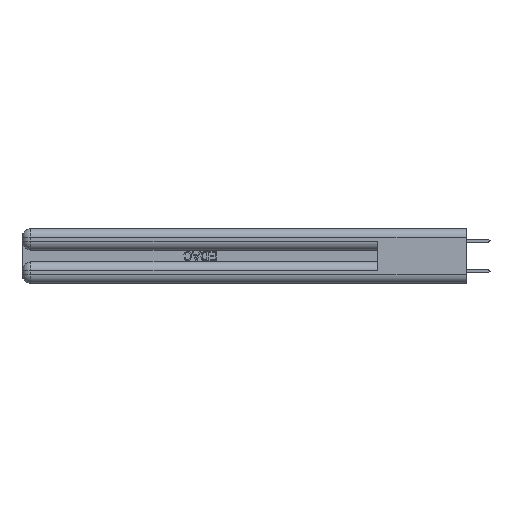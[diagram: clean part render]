
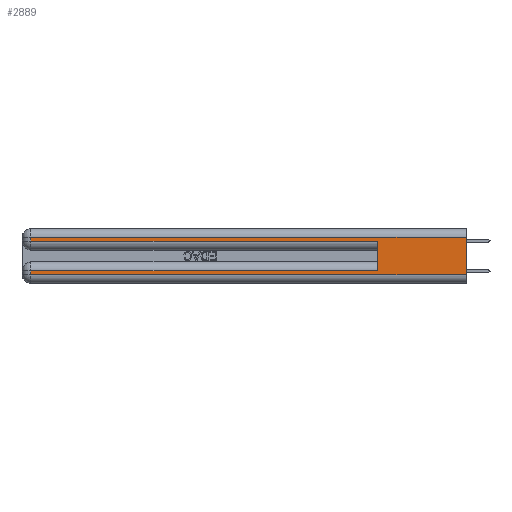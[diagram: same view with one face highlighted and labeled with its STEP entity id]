
A CAD part, left-side view. The second image highlights one B-rep face of the part: STEP entity #2889.
In plain terms, the highlighted planar face has unit normal (-1, 0, 0).
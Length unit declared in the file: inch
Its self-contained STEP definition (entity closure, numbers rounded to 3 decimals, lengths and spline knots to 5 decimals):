
#321 = CARTESIAN_POINT ( 'NONE',  ( 0., 0., 0.31 ) ) ;
#452 = VECTOR ( 'NONE', #42532, 39.37008 ) ;
#540 = DIRECTION ( 'NONE',  ( 0., 0., -1. ) ) ;
#1603 = EDGE_LOOP ( 'NONE', ( #13130, #28414, #34423, #3355, #9886, #20424, #22199, #41420 ) ) ;
#2248 = PLANE ( 'NONE',  #40036 ) ;
#2612 = VECTOR ( 'NONE', #23209, 39.37008 ) ;
#2889 = ADVANCED_FACE ( 'NONE', ( #3151 ), #2248, .F. ) ;
#3112 = EDGE_CURVE ( 'NONE', #30202, #29125, #11382, .T. ) ;
#3151 = FACE_OUTER_BOUND ( 'NONE', #1603, .T. ) ;
#3355 = ORIENTED_EDGE ( 'NONE', *, *, #33864, .T. ) ;
#4314 = DIRECTION ( 'NONE',  ( 0., -1., 0. ) ) ;
#4664 = DIRECTION ( 'NONE',  ( 0., 0., -1. ) ) ;
#4951 = CARTESIAN_POINT ( 'NONE',  ( 0., 2.94, 0.085 ) ) ;
#5555 = DIRECTION ( 'NONE',  ( 0., 0., -1. ) ) ;
#5712 = VERTEX_POINT ( 'NONE', #17757 ) ;
#8087 = VERTEX_POINT ( 'NONE', #321 ) ;
#8635 = VECTOR ( 'NONE', #28004, 39.37008 ) ;
#9085 = CARTESIAN_POINT ( 'NONE',  ( 0., 2.94, 0.285 ) ) ;
#9516 = EDGE_CURVE ( 'NONE', #30202, #16570, #35058, .T. ) ;
#9729 = CARTESIAN_POINT ( 'NONE',  ( 0., 0., 0.31 ) ) ;
#9886 = ORIENTED_EDGE ( 'NONE', *, *, #3112, .F. ) ;
#10216 = VECTOR ( 'NONE', #4664, 39.37008 ) ;
#11249 = LINE ( 'NONE', #18020, #10216 ) ;
#11382 = LINE ( 'NONE', #33048, #2612 ) ;
#13130 = ORIENTED_EDGE ( 'NONE', *, *, #34942, .F. ) ;
#15125 = CARTESIAN_POINT ( 'NONE',  ( 0., 0.6, 0.285 ) ) ;
#15431 = CARTESIAN_POINT ( 'NONE',  ( 0., 0., 0.37 ) ) ;
#16120 = CARTESIAN_POINT ( 'NONE',  ( 0., 2.94, 0.37 ) ) ;
#16570 = VERTEX_POINT ( 'NONE', #4951 ) ;
#16750 = LINE ( 'NONE', #40621, #24503 ) ;
#17039 = LINE ( 'NONE', #39342, #33574 ) ;
#17737 = VECTOR ( 'NONE', #540, 39.37008 ) ;
#17757 = CARTESIAN_POINT ( 'NONE',  ( 0., 2.94, 0.06 ) ) ;
#18020 = CARTESIAN_POINT ( 'NONE',  ( 0., 2.94, 0.37 ) ) ;
#19552 = DIRECTION ( 'NONE',  ( 0., -1., 0. ) ) ;
#20381 = EDGE_CURVE ( 'NONE', #5712, #21275, #17039, .T. ) ;
#20424 = ORIENTED_EDGE ( 'NONE', *, *, #9516, .T. ) ;
#21210 = CARTESIAN_POINT ( 'NONE',  ( 0., 0.6, 0.085 ) ) ;
#21275 = VERTEX_POINT ( 'NONE', #27934 ) ;
#22199 = ORIENTED_EDGE ( 'NONE', *, *, #37454, .T. ) ;
#23209 = DIRECTION ( 'NONE',  ( 0., 0., 1. ) ) ;
#24503 = VECTOR ( 'NONE', #4314, 39.37008 ) ;
#24673 = CARTESIAN_POINT ( 'NONE',  ( 0., 0., 0.085 ) ) ;
#25428 = DIRECTION ( 'NONE',  ( 1., 0., 0. ) ) ;
#26431 = EDGE_CURVE ( 'NONE', #29787, #35978, #26874, .T. ) ;
#26563 = LINE ( 'NONE', #39983, #17737 ) ;
#26874 = LINE ( 'NONE', #16120, #452 ) ;
#27934 = CARTESIAN_POINT ( 'NONE',  ( 0., 0., 0.06 ) ) ;
#28004 = DIRECTION ( 'NONE',  ( 0., 1., 0. ) ) ;
#28414 = ORIENTED_EDGE ( 'NONE', *, *, #41315, .T. ) ;
#29125 = VERTEX_POINT ( 'NONE', #15125 ) ;
#29787 = VERTEX_POINT ( 'NONE', #42049 ) ;
#30202 = VERTEX_POINT ( 'NONE', #21210 ) ;
#33048 = CARTESIAN_POINT ( 'NONE',  ( 0., 0.6, 0.145 ) ) ;
#33574 = VECTOR ( 'NONE', #19552, 39.37008 ) ;
#33864 = EDGE_CURVE ( 'NONE', #35978, #29125, #16750, .T. ) ;
#34423 = ORIENTED_EDGE ( 'NONE', *, *, #26431, .T. ) ;
#34543 = LINE ( 'NONE', #9729, #42267 ) ;
#34942 = EDGE_CURVE ( 'NONE', #8087, #21275, #26563, .T. ) ;
#35058 = LINE ( 'NONE', #24673, #8635 ) ;
#35978 = VERTEX_POINT ( 'NONE', #9085 ) ;
#36216 = DIRECTION ( 'NONE',  ( 0., 1., 0. ) ) ;
#37454 = EDGE_CURVE ( 'NONE', #16570, #5712, #11249, .T. ) ;
#39342 = CARTESIAN_POINT ( 'NONE',  ( 0., 0., 0.06 ) ) ;
#39983 = CARTESIAN_POINT ( 'NONE',  ( 0., 0., 0.37 ) ) ;
#40036 = AXIS2_PLACEMENT_3D ( 'NONE', #15431, #25428, #5555 ) ;
#40621 = CARTESIAN_POINT ( 'NONE',  ( 0., 0., 0.285 ) ) ;
#41315 = EDGE_CURVE ( 'NONE', #8087, #29787, #34543, .T. ) ;
#41420 = ORIENTED_EDGE ( 'NONE', *, *, #20381, .T. ) ;
#42049 = CARTESIAN_POINT ( 'NONE',  ( 0., 2.94, 0.31 ) ) ;
#42267 = VECTOR ( 'NONE', #36216, 39.37008 ) ;
#42532 = DIRECTION ( 'NONE',  ( 0., 0., -1. ) ) ;
